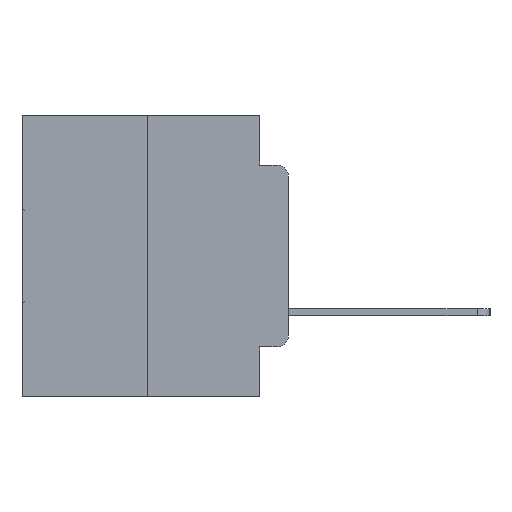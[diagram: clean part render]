
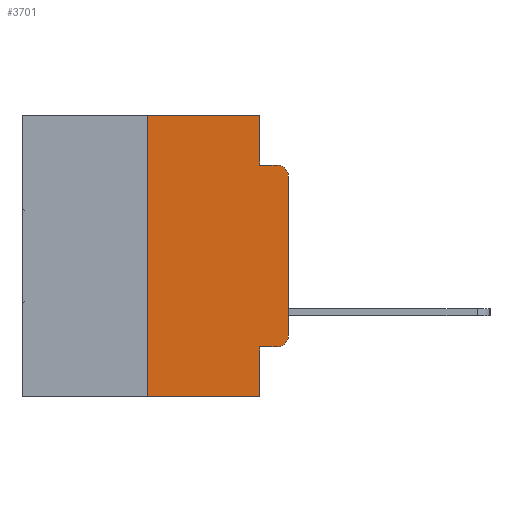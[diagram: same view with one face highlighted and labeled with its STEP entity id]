
A CAD part, left-side view. The second image highlights one B-rep face of the part: STEP entity #3701.
In plain terms, the highlighted planar face has unit normal (-1, 0, 0).
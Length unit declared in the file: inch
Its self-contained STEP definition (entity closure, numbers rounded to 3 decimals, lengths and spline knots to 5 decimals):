
#386 = EDGE_CURVE ( 'NONE', #6460, #20394, #12354, .T. ) ;
#1171 = DIRECTION ( 'NONE',  ( 0., 0., -1. ) ) ;
#1542 = VERTEX_POINT ( 'NONE', #2966 ) ;
#1908 = CARTESIAN_POINT ( 'NONE',  ( 0., 0.25, -0.5 ) ) ;
#1925 = ORIENTED_EDGE ( 'NONE', *, *, #386, .T. ) ;
#2718 = ORIENTED_EDGE ( 'NONE', *, *, #27417, .T. ) ;
#2790 = CARTESIAN_POINT ( 'NONE',  ( 0., 0.02, -0.1085 ) ) ;
#2801 = VECTOR ( 'NONE', #3106, 39.37008 ) ;
#2849 = ORIENTED_EDGE ( 'NONE', *, *, #12375, .T. ) ;
#2966 = CARTESIAN_POINT ( 'NONE',  ( 0., 0.051, -0.0885 ) ) ;
#3106 = DIRECTION ( 'NONE',  ( 0., 0., 1. ) ) ;
#3163 = VECTOR ( 'NONE', #19889, 39.37008 ) ;
#3213 = CARTESIAN_POINT ( 'NONE',  ( 0., 0.25, 0. ) ) ;
#3701 = ADVANCED_FACE ( 'NONE', ( #21589 ), #28290, .F. ) ;
#4058 = LINE ( 'NONE', #5423, #10459 ) ;
#4270 = VERTEX_POINT ( 'NONE', #1908 ) ;
#4293 = CARTESIAN_POINT ( 'NONE',  ( 0., 0.473, -0.5 ) ) ;
#4460 = DIRECTION ( 'NONE',  ( 0., 0., -1. ) ) ;
#5018 = LINE ( 'NONE', #4293, #28622 ) ;
#5020 = ORIENTED_EDGE ( 'NONE', *, *, #25998, .F. ) ;
#5239 = DIRECTION ( 'NONE',  ( 0., 0., -1. ) ) ;
#5423 = CARTESIAN_POINT ( 'NONE',  ( 0., 0.051, 0. ) ) ;
#5564 = EDGE_CURVE ( 'NONE', #23171, #14163, #9070, .T. ) ;
#5961 = VECTOR ( 'NONE', #7373, 39.37008 ) ;
#6018 = CARTESIAN_POINT ( 'NONE',  ( 0., 0.473, 0. ) ) ;
#6460 = VERTEX_POINT ( 'NONE', #9480 ) ;
#6538 = ORIENTED_EDGE ( 'NONE', *, *, #24572, .F. ) ;
#6709 = DIRECTION ( 'NONE',  ( 0., -1., 0. ) ) ;
#6780 = LINE ( 'NONE', #18344, #29493 ) ;
#7214 = DIRECTION ( 'NONE',  ( 1., 0., 0. ) ) ;
#7337 = CARTESIAN_POINT ( 'NONE',  ( 0., 0.473, 0. ) ) ;
#7373 = DIRECTION ( 'NONE',  ( 0., 0., 1. ) ) ;
#8537 = CIRCLE ( 'NONE', #9946, 0.02 ) ;
#8661 = CARTESIAN_POINT ( 'NONE',  ( 0., 0.051, 0. ) ) ;
#8750 = VECTOR ( 'NONE', #4460, 39.37008 ) ;
#9070 = LINE ( 'NONE', #7337, #15333 ) ;
#9480 = CARTESIAN_POINT ( 'NONE',  ( 0., 0., -0.3915 ) ) ;
#9946 = AXIS2_PLACEMENT_3D ( 'NONE', #28827, #15571, #1171 ) ;
#10459 = VECTOR ( 'NONE', #28219, 39.37008 ) ;
#12315 = CARTESIAN_POINT ( 'NONE',  ( 0., 0.02, -0.0885 ) ) ;
#12354 = LINE ( 'NONE', #18444, #5961 ) ;
#12375 = EDGE_CURVE ( 'NONE', #17516, #6460, #8537, .T. ) ;
#12454 = CARTESIAN_POINT ( 'NONE',  ( 0., 0.051, -0.4115 ) ) ;
#12656 = ORIENTED_EDGE ( 'NONE', *, *, #15505, .T. ) ;
#14035 = VERTEX_POINT ( 'NONE', #12315 ) ;
#14163 = VERTEX_POINT ( 'NONE', #8661 ) ;
#15033 = CARTESIAN_POINT ( 'NONE',  ( 0., 0.25, 0. ) ) ;
#15039 = LINE ( 'NONE', #16337, #8750 ) ;
#15333 = VECTOR ( 'NONE', #19109, 39.37008 ) ;
#15505 = EDGE_CURVE ( 'NONE', #17626, #17516, #21933, .T. ) ;
#15571 = DIRECTION ( 'NONE',  ( -1., 0., 0. ) ) ;
#16337 = CARTESIAN_POINT ( 'NONE',  ( 0., 0.051, 0. ) ) ;
#17116 = CARTESIAN_POINT ( 'NONE',  ( 0., 0.051, -0.5 ) ) ;
#17516 = VERTEX_POINT ( 'NONE', #23647 ) ;
#17626 = VERTEX_POINT ( 'NONE', #12454 ) ;
#18030 = ORIENTED_EDGE ( 'NONE', *, *, #27786, .T. ) ;
#18118 = CARTESIAN_POINT ( 'NONE',  ( 0., 0., -0.1085 ) ) ;
#18344 = CARTESIAN_POINT ( 'NONE',  ( 0., 0.051, -0.0885 ) ) ;
#18444 = CARTESIAN_POINT ( 'NONE',  ( 0., 0., 0. ) ) ;
#18645 = EDGE_CURVE ( 'NONE', #17626, #20011, #4058, .T. ) ;
#18803 = AXIS2_PLACEMENT_3D ( 'NONE', #2790, #19433, #5239 ) ;
#19109 = DIRECTION ( 'NONE',  ( 0., -1., 0. ) ) ;
#19433 = DIRECTION ( 'NONE',  ( -1., 0., 0. ) ) ;
#19889 = DIRECTION ( 'NONE',  ( 0., -1., 0. ) ) ;
#20011 = VERTEX_POINT ( 'NONE', #17116 ) ;
#20394 = VERTEX_POINT ( 'NONE', #18118 ) ;
#20619 = ORIENTED_EDGE ( 'NONE', *, *, #18645, .F. ) ;
#21589 = FACE_OUTER_BOUND ( 'NONE', #23759, .T. ) ;
#21630 = LINE ( 'NONE', #15033, #2801 ) ;
#21933 = LINE ( 'NONE', #22189, #3163 ) ;
#22189 = CARTESIAN_POINT ( 'NONE',  ( 0., 0.051, -0.4115 ) ) ;
#23110 = EDGE_CURVE ( 'NONE', #4270, #23171, #21630, .T. ) ;
#23171 = VERTEX_POINT ( 'NONE', #3213 ) ;
#23647 = CARTESIAN_POINT ( 'NONE',  ( 0., 0.02, -0.4115 ) ) ;
#23759 = EDGE_LOOP ( 'NONE', ( #1925, #2718, #5020, #6538, #24969, #25631, #18030, #20619, #12656, #2849 ) ) ;
#24572 = EDGE_CURVE ( 'NONE', #14163, #1542, #15039, .T. ) ;
#24969 = ORIENTED_EDGE ( 'NONE', *, *, #5564, .F. ) ;
#25631 = ORIENTED_EDGE ( 'NONE', *, *, #23110, .F. ) ;
#25998 = EDGE_CURVE ( 'NONE', #1542, #14035, #6780, .T. ) ;
#26342 = DIRECTION ( 'NONE',  ( 0., 0., -1. ) ) ;
#26415 = CIRCLE ( 'NONE', #18803, 0.02 ) ;
#27417 = EDGE_CURVE ( 'NONE', #20394, #14035, #26415, .T. ) ;
#27786 = EDGE_CURVE ( 'NONE', #4270, #20011, #5018, .T. ) ;
#28219 = DIRECTION ( 'NONE',  ( 0., 0., -1. ) ) ;
#28290 = PLANE ( 'NONE',  #29307 ) ;
#28622 = VECTOR ( 'NONE', #6709, 39.37008 ) ;
#28827 = CARTESIAN_POINT ( 'NONE',  ( 0., 0.02, -0.3915 ) ) ;
#29299 = DIRECTION ( 'NONE',  ( 0., -1., 0. ) ) ;
#29307 = AXIS2_PLACEMENT_3D ( 'NONE', #6018, #7214, #26342 ) ;
#29493 = VECTOR ( 'NONE', #29299, 39.37008 ) ;
